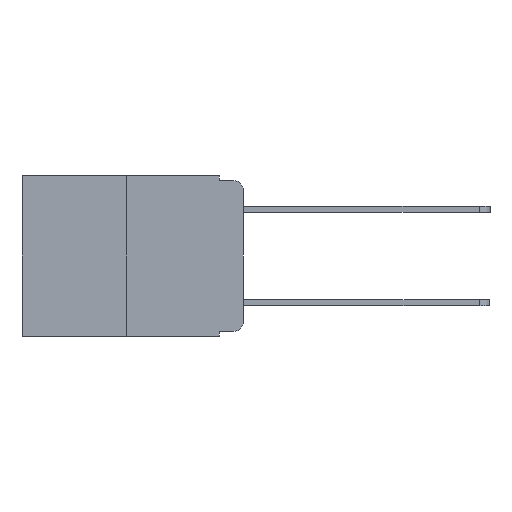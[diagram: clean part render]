
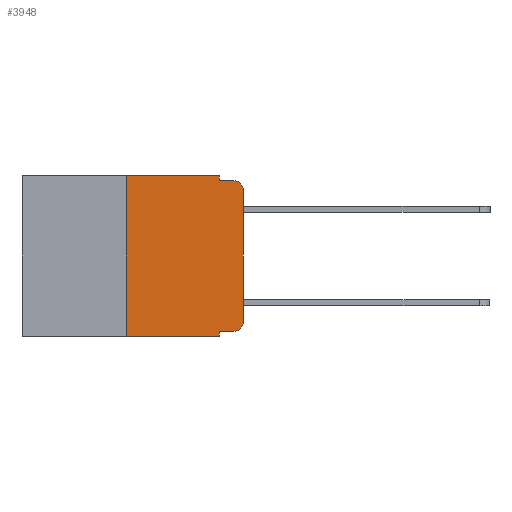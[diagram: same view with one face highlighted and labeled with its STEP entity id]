
A CAD part, left-side view. The second image highlights one B-rep face of the part: STEP entity #3948.
In plain terms, the highlighted planar face has unit normal (-1, 0, 0).
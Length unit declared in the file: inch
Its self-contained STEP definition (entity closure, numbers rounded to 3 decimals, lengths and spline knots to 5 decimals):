
#164 = LINE ( 'NONE', #4236, #1782 ) ;
#258 = VECTOR ( 'NONE', #7354, 39.37008 ) ;
#358 = DIRECTION ( 'NONE',  ( -1., 0., 0. ) ) ;
#423 = DIRECTION ( 'NONE',  ( 0., 0., -1. ) ) ;
#505 = PLANE ( 'NONE',  #5968 ) ;
#726 = VERTEX_POINT ( 'NONE', #4284 ) ;
#731 = CARTESIAN_POINT ( 'NONE',  ( 0., 0., 0. ) ) ;
#783 = DIRECTION ( 'NONE',  ( 0., 0., 1. ) ) ;
#1037 = CARTESIAN_POINT ( 'NONE',  ( 0., 0.051, -0.01 ) ) ;
#1079 = EDGE_CURVE ( 'NONE', #7986, #1600, #1983, .T. ) ;
#1214 = CARTESIAN_POINT ( 'NONE',  ( 0., 0.02, -0.01 ) ) ;
#1334 = CARTESIAN_POINT ( 'NONE',  ( 0., 0.02, -0.03 ) ) ;
#1600 = VERTEX_POINT ( 'NONE', #2622 ) ;
#1719 = ORIENTED_EDGE ( 'NONE', *, *, #6052, .F. ) ;
#1782 = VECTOR ( 'NONE', #7104, 39.37008 ) ;
#1855 = VERTEX_POINT ( 'NONE', #5534 ) ;
#1983 = LINE ( 'NONE', #8336, #9370 ) ;
#2364 = ORIENTED_EDGE ( 'NONE', *, *, #4505, .T. ) ;
#2377 = EDGE_LOOP ( 'NONE', ( #3231, #5751, #5741, #6085, #3345, #1719, #4883, #4518, #6725, #2364 ) ) ;
#2429 = DIRECTION ( 'NONE',  ( 0., 0., -1. ) ) ;
#2463 = LINE ( 'NONE', #8393, #6064 ) ;
#2531 = CARTESIAN_POINT ( 'NONE',  ( 0., 0.051, 0. ) ) ;
#2622 = CARTESIAN_POINT ( 'NONE',  ( 0., 0.051, -0.343 ) ) ;
#2681 = DIRECTION ( 'NONE',  ( 0., -1., 0. ) ) ;
#2737 = LINE ( 'NONE', #3276, #4251 ) ;
#2807 = LINE ( 'NONE', #5369, #8355 ) ;
#3045 = VECTOR ( 'NONE', #2429, 39.37008 ) ;
#3136 = CARTESIAN_POINT ( 'NONE',  ( 0., 0.473, 0. ) ) ;
#3231 = ORIENTED_EDGE ( 'NONE', *, *, #7855, .T. ) ;
#3276 = CARTESIAN_POINT ( 'NONE',  ( 0., 0.051, -0.333 ) ) ;
#3345 = ORIENTED_EDGE ( 'NONE', *, *, #7470, .F. ) ;
#3419 = DIRECTION ( 'NONE',  ( 0., -1., 0. ) ) ;
#3428 = LINE ( 'NONE', #731, #8925 ) ;
#3525 = AXIS2_PLACEMENT_3D ( 'NONE', #8547, #7988, #5571 ) ;
#3567 = CARTESIAN_POINT ( 'NONE',  ( 0., 0.02, -0.333 ) ) ;
#3948 = ADVANCED_FACE ( 'NONE', ( #6652 ), #505, .F. ) ;
#4119 = CIRCLE ( 'NONE', #3525, 0.02 ) ;
#4236 = CARTESIAN_POINT ( 'NONE',  ( 0., 0.25, 0. ) ) ;
#4251 = VECTOR ( 'NONE', #2681, 39.37008 ) ;
#4284 = CARTESIAN_POINT ( 'NONE',  ( 0., 0.25, 0. ) ) ;
#4319 = LINE ( 'NONE', #7730, #258 ) ;
#4505 = EDGE_CURVE ( 'NONE', #7358, #1855, #4119, .T. ) ;
#4518 = ORIENTED_EDGE ( 'NONE', *, *, #5548, .F. ) ;
#4883 = ORIENTED_EDGE ( 'NONE', *, *, #1079, .T. ) ;
#5025 = EDGE_CURVE ( 'NONE', #7603, #7358, #2737, .T. ) ;
#5314 = VERTEX_POINT ( 'NONE', #7536 ) ;
#5369 = CARTESIAN_POINT ( 'NONE',  ( 0., 0.051, -0.01 ) ) ;
#5529 = CARTESIAN_POINT ( 'NONE',  ( 0., 0.25, -0.343 ) ) ;
#5534 = CARTESIAN_POINT ( 'NONE',  ( 0., 0., -0.313 ) ) ;
#5538 = DIRECTION ( 'NONE',  ( 0., 0., -1. ) ) ;
#5548 = EDGE_CURVE ( 'NONE', #7603, #1600, #2463, .T. ) ;
#5571 = DIRECTION ( 'NONE',  ( 0., 0., -1. ) ) ;
#5741 = ORIENTED_EDGE ( 'NONE', *, *, #6947, .F. ) ;
#5751 = ORIENTED_EDGE ( 'NONE', *, *, #7408, .T. ) ;
#5920 = AXIS2_PLACEMENT_3D ( 'NONE', #1334, #358, #423 ) ;
#5968 = AXIS2_PLACEMENT_3D ( 'NONE', #3136, #7346, #5538 ) ;
#6052 = EDGE_CURVE ( 'NONE', #7986, #726, #164, .T. ) ;
#6064 = VECTOR ( 'NONE', #7614, 39.37008 ) ;
#6085 = ORIENTED_EDGE ( 'NONE', *, *, #6552, .F. ) ;
#6258 = VERTEX_POINT ( 'NONE', #1037 ) ;
#6552 = EDGE_CURVE ( 'NONE', #5314, #6258, #8584, .T. ) ;
#6652 = FACE_OUTER_BOUND ( 'NONE', #2377, .T. ) ;
#6725 = ORIENTED_EDGE ( 'NONE', *, *, #5025, .T. ) ;
#6947 = EDGE_CURVE ( 'NONE', #6258, #7210, #2807, .T. ) ;
#7104 = DIRECTION ( 'NONE',  ( 0., 0., 1. ) ) ;
#7201 = CARTESIAN_POINT ( 'NONE',  ( 0., 0.051, -0.333 ) ) ;
#7210 = VERTEX_POINT ( 'NONE', #1214 ) ;
#7346 = DIRECTION ( 'NONE',  ( 1., 0., 0. ) ) ;
#7354 = DIRECTION ( 'NONE',  ( 0., -1., 0. ) ) ;
#7358 = VERTEX_POINT ( 'NONE', #3567 ) ;
#7408 = EDGE_CURVE ( 'NONE', #8417, #7210, #8781, .T. ) ;
#7470 = EDGE_CURVE ( 'NONE', #726, #5314, #4319, .T. ) ;
#7536 = CARTESIAN_POINT ( 'NONE',  ( 0., 0.051, 0. ) ) ;
#7603 = VERTEX_POINT ( 'NONE', #7201 ) ;
#7614 = DIRECTION ( 'NONE',  ( 0., 0., -1. ) ) ;
#7730 = CARTESIAN_POINT ( 'NONE',  ( 0., 0.473, 0. ) ) ;
#7746 = DIRECTION ( 'NONE',  ( 0., -1., 0. ) ) ;
#7855 = EDGE_CURVE ( 'NONE', #1855, #8417, #3428, .T. ) ;
#7986 = VERTEX_POINT ( 'NONE', #5529 ) ;
#7988 = DIRECTION ( 'NONE',  ( -1., 0., 0. ) ) ;
#8336 = CARTESIAN_POINT ( 'NONE',  ( 0., 0.473, -0.343 ) ) ;
#8355 = VECTOR ( 'NONE', #7746, 39.37008 ) ;
#8393 = CARTESIAN_POINT ( 'NONE',  ( 0., 0.051, 0. ) ) ;
#8417 = VERTEX_POINT ( 'NONE', #9086 ) ;
#8547 = CARTESIAN_POINT ( 'NONE',  ( 0., 0.02, -0.313 ) ) ;
#8584 = LINE ( 'NONE', #2531, #3045 ) ;
#8781 = CIRCLE ( 'NONE', #5920, 0.02 ) ;
#8925 = VECTOR ( 'NONE', #783, 39.37008 ) ;
#9086 = CARTESIAN_POINT ( 'NONE',  ( 0., 0., -0.03 ) ) ;
#9370 = VECTOR ( 'NONE', #3419, 39.37008 ) ;
